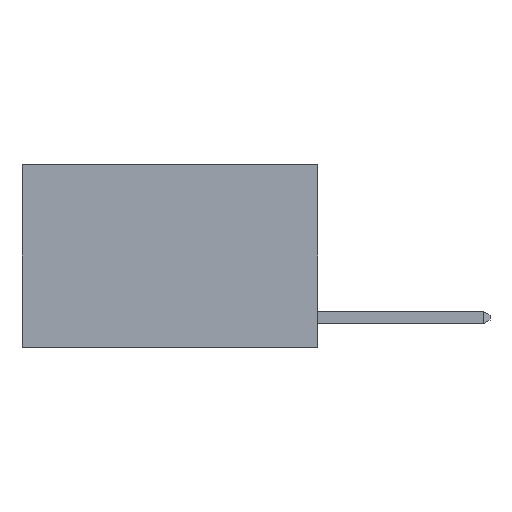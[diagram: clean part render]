
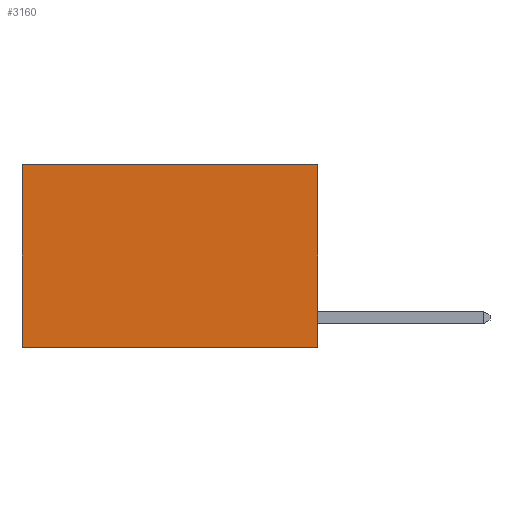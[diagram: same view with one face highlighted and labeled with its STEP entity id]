
A CAD part, left-side view. The second image highlights one B-rep face of the part: STEP entity #3160.
In plain terms, the highlighted planar face has unit normal (-1, 0, 0).
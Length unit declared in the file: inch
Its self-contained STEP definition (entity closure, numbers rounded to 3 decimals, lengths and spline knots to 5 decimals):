
#399 = VECTOR ( 'NONE', #1467, 39.37008 ) ;
#405 = VERTEX_POINT ( 'NONE', #9339 ) ;
#984 = ORIENTED_EDGE ( 'NONE', *, *, #3535, .T. ) ;
#1467 = DIRECTION ( 'NONE',  ( 0., 0., -1. ) ) ;
#2216 = LINE ( 'NONE', #6101, #7732 ) ;
#2678 = EDGE_CURVE ( 'NONE', #5377, #8132, #6268, .T. ) ;
#3160 = ADVANCED_FACE ( 'NONE', ( #5255 ), #7088, .F. ) ;
#3231 = CARTESIAN_POINT ( 'NONE',  ( 0.2625, 0., 0. ) ) ;
#3302 = EDGE_LOOP ( 'NONE', ( #984, #5602, #6618, #5762 ) ) ;
#3535 = EDGE_CURVE ( 'NONE', #8132, #5453, #2216, .T. ) ;
#3930 = VECTOR ( 'NONE', #7737, 39.37008 ) ;
#4197 = LINE ( 'NONE', #7747, #3930 ) ;
#4217 = EDGE_CURVE ( 'NONE', #5377, #405, #5120, .T. ) ;
#4737 = VECTOR ( 'NONE', #5452, 39.37008 ) ;
#5120 = LINE ( 'NONE', #3231, #399 ) ;
#5255 = FACE_OUTER_BOUND ( 'NONE', #3302, .T. ) ;
#5377 = VERTEX_POINT ( 'NONE', #6174 ) ;
#5430 = CARTESIAN_POINT ( 'NONE',  ( 0.2625, 0.6, -0.37 ) ) ;
#5452 = DIRECTION ( 'NONE',  ( 0., 1., 0. ) ) ;
#5453 = VERTEX_POINT ( 'NONE', #5430 ) ;
#5521 = AXIS2_PLACEMENT_3D ( 'NONE', #5946, #5561, #9086 ) ;
#5561 = DIRECTION ( 'NONE',  ( 1., 0., 0. ) ) ;
#5602 = ORIENTED_EDGE ( 'NONE', *, *, #8398, .F. ) ;
#5762 = ORIENTED_EDGE ( 'NONE', *, *, #2678, .T. ) ;
#5946 = CARTESIAN_POINT ( 'NONE',  ( 0.2625, 0., 0. ) ) ;
#6101 = CARTESIAN_POINT ( 'NONE',  ( 0.2625, 0.6, 0. ) ) ;
#6174 = CARTESIAN_POINT ( 'NONE',  ( 0.2625, 0., 0. ) ) ;
#6268 = LINE ( 'NONE', #7967, #4737 ) ;
#6612 = DIRECTION ( 'NONE',  ( 0., 0., -1. ) ) ;
#6618 = ORIENTED_EDGE ( 'NONE', *, *, #4217, .F. ) ;
#7088 = PLANE ( 'NONE',  #5521 ) ;
#7732 = VECTOR ( 'NONE', #6612, 39.37008 ) ;
#7737 = DIRECTION ( 'NONE',  ( 0., 1., 0. ) ) ;
#7747 = CARTESIAN_POINT ( 'NONE',  ( 0.2625, 0., -0.37 ) ) ;
#7967 = CARTESIAN_POINT ( 'NONE',  ( 0.2625, 0., 0. ) ) ;
#8132 = VERTEX_POINT ( 'NONE', #9315 ) ;
#8398 = EDGE_CURVE ( 'NONE', #405, #5453, #4197, .T. ) ;
#9086 = DIRECTION ( 'NONE',  ( 0., 0., -1. ) ) ;
#9315 = CARTESIAN_POINT ( 'NONE',  ( 0.2625, 0.6, 0. ) ) ;
#9339 = CARTESIAN_POINT ( 'NONE',  ( 0.2625, 0., -0.37 ) ) ;
